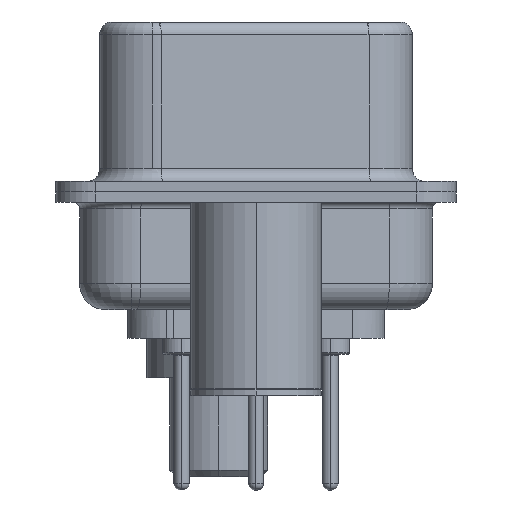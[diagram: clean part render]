
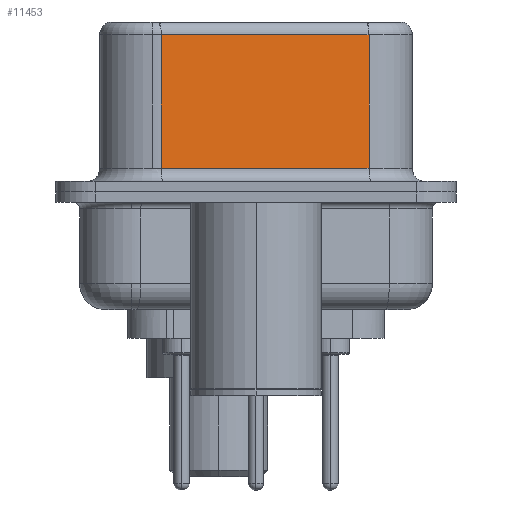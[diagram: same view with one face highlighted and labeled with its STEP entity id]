
A CAD part, left-side view. The second image highlights one B-rep face of the part: STEP entity #11453.
In plain terms, the highlighted planar face has unit normal (-0.985, -0.174, 0).
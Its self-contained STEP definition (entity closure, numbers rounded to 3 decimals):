
#160 = VECTOR ( 'NONE', #3429, 1000. ) ;
#888 = VERTEX_POINT ( 'NONE', #10872 ) ;
#1300 = VERTEX_POINT ( 'NONE', #29668 ) ;
#1671 = PLANE ( 'NONE',  #10438 ) ;
#1970 = FACE_OUTER_BOUND ( 'NONE', #26777, .T. ) ;
#3429 = DIRECTION ( 'NONE',  ( 0., 0., -1. ) ) ;
#4114 = CARTESIAN_POINT ( 'NONE',  ( 5.132, -4.322, 6.52 ) ) ;
#4227 = DIRECTION ( 'NONE',  ( 0.985, 0.174, 0. ) ) ;
#4628 = VERTEX_POINT ( 'NONE', #15063 ) ;
#7450 = VECTOR ( 'NONE', #7900, 1000. ) ;
#7597 = ORIENTED_EDGE ( 'NONE', *, *, #22145, .F. ) ;
#7900 = DIRECTION ( 'NONE',  ( 0.174, -0.985, 0. ) ) ;
#9487 = CARTESIAN_POINT ( 'NONE',  ( 5.132, -4.322, 6.52 ) ) ;
#10438 = AXIS2_PLACEMENT_3D ( 'NONE', #4114, #4227, #21839 ) ;
#10872 = CARTESIAN_POINT ( 'NONE',  ( 3.73, 3.628, 6.02 ) ) ;
#11453 = ADVANCED_FACE ( 'NONE', ( #1970 ), #1671, .F. ) ;
#12851 = LINE ( 'NONE', #9487, #25436 ) ;
#13002 = CARTESIAN_POINT ( 'NONE',  ( 5.132, -4.322, 0.9 ) ) ;
#15063 = CARTESIAN_POINT ( 'NONE',  ( 5.132, -4.322, 0.9 ) ) ;
#16579 = VERTEX_POINT ( 'NONE', #22288 ) ;
#16724 = LINE ( 'NONE', #20674, #21821 ) ;
#16974 = DIRECTION ( 'NONE',  ( 0., 0., -1. ) ) ;
#20094 = LINE ( 'NONE', #13002, #7450 ) ;
#20167 = EDGE_CURVE ( 'NONE', #888, #16579, #20283, .T. ) ;
#20283 = LINE ( 'NONE', #21064, #160 ) ;
#20317 = ORIENTED_EDGE ( 'NONE', *, *, #27549, .T. ) ;
#20674 = CARTESIAN_POINT ( 'NONE',  ( 5.132, -4.322, 6.02 ) ) ;
#21064 = CARTESIAN_POINT ( 'NONE',  ( 3.73, 3.628, 6.52 ) ) ;
#21821 = VECTOR ( 'NONE', #23189, 1000. ) ;
#21839 = DIRECTION ( 'NONE',  ( -0.174, 0.985, 0. ) ) ;
#22145 = EDGE_CURVE ( 'NONE', #1300, #4628, #12851, .T. ) ;
#22288 = CARTESIAN_POINT ( 'NONE',  ( 3.73, 3.628, 0.9 ) ) ;
#23189 = DIRECTION ( 'NONE',  ( -0.174, 0.985, 0. ) ) ;
#23209 = EDGE_CURVE ( 'NONE', #1300, #888, #16724, .T. ) ;
#25436 = VECTOR ( 'NONE', #16974, 1000. ) ;
#25667 = ORIENTED_EDGE ( 'NONE', *, *, #20167, .T. ) ;
#26777 = EDGE_LOOP ( 'NONE', ( #7597, #28032, #25667, #20317 ) ) ;
#27549 = EDGE_CURVE ( 'NONE', #16579, #4628, #20094, .T. ) ;
#28032 = ORIENTED_EDGE ( 'NONE', *, *, #23209, .T. ) ;
#29668 = CARTESIAN_POINT ( 'NONE',  ( 5.132, -4.322, 6.02 ) ) ;
